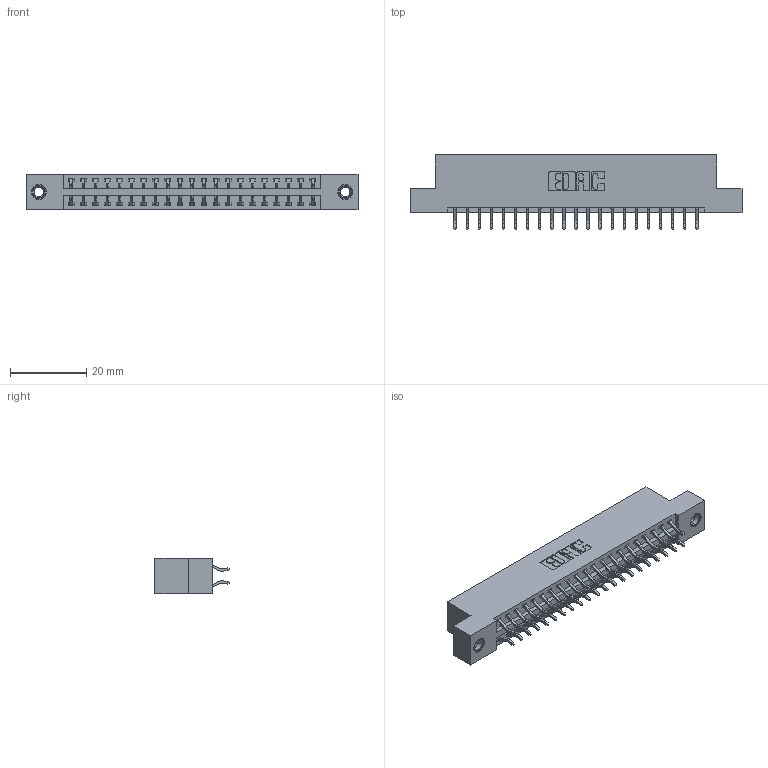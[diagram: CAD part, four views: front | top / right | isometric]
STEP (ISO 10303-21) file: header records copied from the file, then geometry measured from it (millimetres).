
FILE_DESCRIPTION (( 'STEP AP203' ), '1' );
FILE_NAME ('346-042-556-207.STEP', '2022-05-20T05:07:43', ( '' ), ( '' ), 'SwSTEP 2.0', 'SolidWorks 2020', '' );
FILE_SCHEMA (( 'CONFIG_CONTROL_DESIGN' ));
Length unit declared in the file: inch
Products named in the file (4): 345-250-001_345-250-005-103; 346-042-556-207; 346 Part_Flush Mounting Lugs - 0.156 Dia-TI; 345-292-001_556 Tail
Assembly tree (45 placements, depth 2):
  346-042-556-207
    346 Part_Flush Mounting Lugs - 0.156 Dia-TI
    345-292-001_556 Tail  x42
    345-250-001_345-250-005-103  x2
Bounding box: 87.25 x 19.57 x 9.4 mm (x, y, z)
Volume: 8329.6 mm3; surface area: 11114.2 mm2
Topology: 45 solids, 45 shells, 2618 faces, 7731 edges, 5090 vertices
Faces by surface type: plane 1746, cylinder 856, cone 12, torus 4
Entity records: 17938 total; most frequent: CARTESIAN_POINT 2983, ORIENTED_EDGE 2898, DIRECTION 2695, EDGE_CURVE 1449, VECTOR 1205, LINE 1205, VERTEX_POINT 960, AXIS2_PLACEMENT_3D 745
